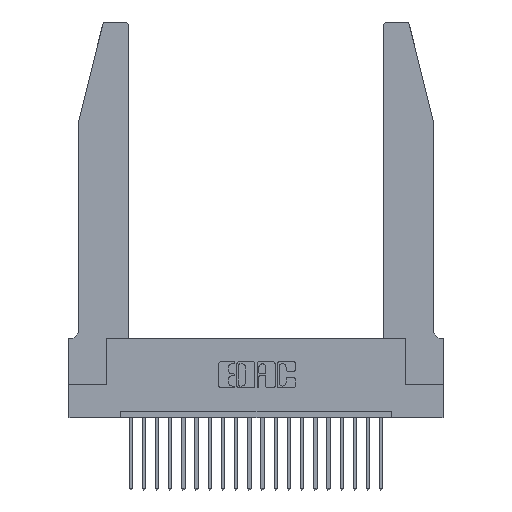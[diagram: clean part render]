
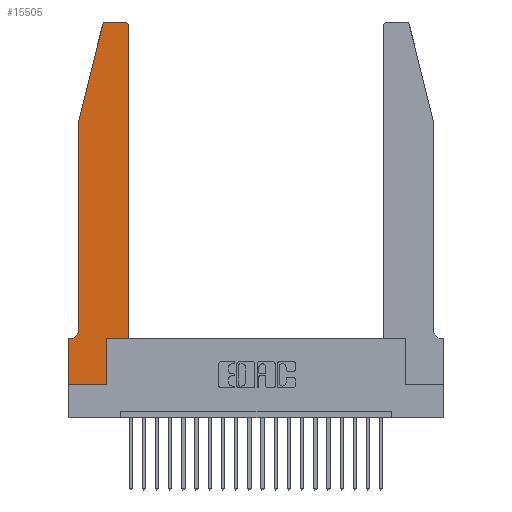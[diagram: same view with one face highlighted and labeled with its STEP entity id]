
A CAD part, top view. The second image highlights one B-rep face of the part: STEP entity #15505.
In plain terms, the highlighted planar face has unit normal (0, 0, 1).
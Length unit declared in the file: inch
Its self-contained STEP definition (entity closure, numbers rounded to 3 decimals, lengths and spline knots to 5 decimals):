
#384 = DIRECTION ( 'NONE',  ( 0., -1., 0. ) ) ;
#406 = CARTESIAN_POINT ( 'NONE',  ( 0.2865, 0.35, 0.37 ) ) ;
#459 = EDGE_CURVE ( 'NONE', #22154, #4561, #3042, .T. ) ;
#637 = VERTEX_POINT ( 'NONE', #22214 ) ;
#841 = DIRECTION ( 'NONE',  ( 0., 0., 1. ) ) ;
#859 = AXIS2_PLACEMENT_3D ( 'NONE', #9379, #18287, #14597 ) ;
#917 = LINE ( 'NONE', #16121, #5352 ) ;
#1115 = LINE ( 'NONE', #6420, #7210 ) ;
#1199 = VERTEX_POINT ( 'NONE', #1847 ) ;
#1201 = ORIENTED_EDGE ( 'NONE', *, *, #12036, .T. ) ;
#1287 = ORIENTED_EDGE ( 'NONE', *, *, #14387, .T. ) ;
#1458 = DIRECTION ( 'NONE',  ( 1., 0., 0. ) ) ;
#1847 = CARTESIAN_POINT ( 'NONE',  ( 0.25487, 2.72718, 0.37 ) ) ;
#2315 = LINE ( 'NONE', #10882, #7547 ) ;
#2342 = VECTOR ( 'NONE', #6219, 39.37008 ) ;
#2479 = ORIENTED_EDGE ( 'NONE', *, *, #12686, .T. ) ;
#2658 = PLANE ( 'NONE',  #859 ) ;
#2955 = CARTESIAN_POINT ( 'NONE',  ( 0.4505, 0.35, 0.37 ) ) ;
#3042 = CIRCLE ( 'NONE', #22489, 0.03 ) ;
#3784 = ORIENTED_EDGE ( 'NONE', *, *, #10910, .T. ) ;
#3871 = VECTOR ( 'NONE', #19753, 39.37008 ) ;
#4238 = DIRECTION ( 'NONE',  ( 0., 1., 0. ) ) ;
#4561 = VERTEX_POINT ( 'NONE', #5781 ) ;
#4858 = VERTEX_POINT ( 'NONE', #21135 ) ;
#4943 = CARTESIAN_POINT ( 'NONE',  ( 0., 0., 0.37 ) ) ;
#4972 = DIRECTION ( 'NONE',  ( 0., 0., -1. ) ) ;
#5352 = VECTOR ( 'NONE', #5683, 39.37008 ) ;
#5404 = DIRECTION ( 'NONE',  ( 1., 0., 0. ) ) ;
#5683 = DIRECTION ( 'NONE',  ( -1., 0., 0. ) ) ;
#5719 = DIRECTION ( 'NONE',  ( 0., 0., 1. ) ) ;
#5781 = CARTESIAN_POINT ( 'NONE',  ( 0.4205, 2.75, 0.37 ) ) ;
#6219 = DIRECTION ( 'NONE',  ( 0., 1., 0. ) ) ;
#6420 = CARTESIAN_POINT ( 'NONE',  ( 0.0755, 2., 0.37 ) ) ;
#6532 = CARTESIAN_POINT ( 'NONE',  ( 0.0055, 0.42, 0.37 ) ) ;
#6735 = VECTOR ( 'NONE', #15798, 39.37008 ) ;
#6936 = EDGE_LOOP ( 'NONE', ( #21626, #1287, #1201, #2479, #14237, #21215, #8851, #3784, #11125, #22543, #9801, #12540 ) ) ;
#7210 = VECTOR ( 'NONE', #9881, 39.37008 ) ;
#7235 = LINE ( 'NONE', #4943, #19530 ) ;
#7547 = VECTOR ( 'NONE', #384, 39.37008 ) ;
#7924 = AXIS2_PLACEMENT_3D ( 'NONE', #6532, #4972, #8370 ) ;
#8034 = CARTESIAN_POINT ( 'NONE',  ( 0.4505, 2.72, 0.37 ) ) ;
#8054 = LINE ( 'NONE', #12281, #20352 ) ;
#8370 = DIRECTION ( 'NONE',  ( -1., 0., 0. ) ) ;
#8851 = ORIENTED_EDGE ( 'NONE', *, *, #16362, .T. ) ;
#9214 = EDGE_CURVE ( 'NONE', #21976, #17296, #9794, .T. ) ;
#9379 = CARTESIAN_POINT ( 'NONE',  ( 0., 0.35, 0.37 ) ) ;
#9600 = EDGE_CURVE ( 'NONE', #4858, #22154, #19035, .T. ) ;
#9701 = VERTEX_POINT ( 'NONE', #17264 ) ;
#9794 = LINE ( 'NONE', #14710, #14934 ) ;
#9801 = ORIENTED_EDGE ( 'NONE', *, *, #9600, .T. ) ;
#9860 = CARTESIAN_POINT ( 'NONE',  ( 0.0755, 0.42, 0.37 ) ) ;
#9881 = DIRECTION ( 'NONE',  ( -0.239, -0.971, 0. ) ) ;
#9922 = EDGE_CURVE ( 'NONE', #14641, #637, #19582, .T. ) ;
#10882 = CARTESIAN_POINT ( 'NONE',  ( 0., 0., 0.37 ) ) ;
#10886 = CARTESIAN_POINT ( 'NONE',  ( 0.2865, 0., 0.37 ) ) ;
#10910 = EDGE_CURVE ( 'NONE', #22359, #21976, #7235, .T. ) ;
#11125 = ORIENTED_EDGE ( 'NONE', *, *, #9214, .T. ) ;
#11634 = AXIS2_PLACEMENT_3D ( 'NONE', #16158, #5719, #17941 ) ;
#11737 = EDGE_CURVE ( 'NONE', #17296, #4858, #8054, .T. ) ;
#12006 = CARTESIAN_POINT ( 'NONE',  ( 0.0755, 2., 0.37 ) ) ;
#12036 = EDGE_CURVE ( 'NONE', #1199, #12834, #1115, .T. ) ;
#12209 = CARTESIAN_POINT ( 'NONE',  ( 0., 0., 0.37 ) ) ;
#12281 = CARTESIAN_POINT ( 'NONE',  ( 0.4505, 0.35, 0.37 ) ) ;
#12540 = ORIENTED_EDGE ( 'NONE', *, *, #459, .T. ) ;
#12686 = EDGE_CURVE ( 'NONE', #12834, #14280, #17003, .T. ) ;
#12834 = VERTEX_POINT ( 'NONE', #12006 ) ;
#12839 = CARTESIAN_POINT ( 'NONE',  ( 0.0755, 2., 0.37 ) ) ;
#14237 = ORIENTED_EDGE ( 'NONE', *, *, #21799, .T. ) ;
#14280 = VERTEX_POINT ( 'NONE', #9860 ) ;
#14384 = FACE_OUTER_BOUND ( 'NONE', #6936, .T. ) ;
#14387 = EDGE_CURVE ( 'NONE', #9701, #1199, #15268, .T. ) ;
#14597 = DIRECTION ( 'NONE',  ( 1., 0., 0. ) ) ;
#14641 = VERTEX_POINT ( 'NONE', #16525 ) ;
#14710 = CARTESIAN_POINT ( 'NONE',  ( 0.2865, 0.35, 0.37 ) ) ;
#14934 = VECTOR ( 'NONE', #4238, 39.37008 ) ;
#15268 = CIRCLE ( 'NONE', #11634, 0.03 ) ;
#15505 = ADVANCED_FACE ( 'NONE', ( #14384 ), #2658, .T. ) ;
#15798 = DIRECTION ( 'NONE',  ( -1., 0., 0. ) ) ;
#15880 = CARTESIAN_POINT ( 'NONE',  ( 0.0755, 0.35, 0.37 ) ) ;
#16059 = EDGE_CURVE ( 'NONE', #4561, #9701, #917, .T. ) ;
#16121 = CARTESIAN_POINT ( 'NONE',  ( 0.2605, 2.75, 0.37 ) ) ;
#16158 = CARTESIAN_POINT ( 'NONE',  ( 0.284, 2.72, 0.37 ) ) ;
#16362 = EDGE_CURVE ( 'NONE', #637, #22359, #2315, .T. ) ;
#16525 = CARTESIAN_POINT ( 'NONE',  ( 0.0055, 0.35, 0.37 ) ) ;
#16794 = CIRCLE ( 'NONE', #7924, 0.07 ) ;
#17003 = LINE ( 'NONE', #12839, #3871 ) ;
#17264 = CARTESIAN_POINT ( 'NONE',  ( 0.284, 2.75, 0.37 ) ) ;
#17296 = VERTEX_POINT ( 'NONE', #406 ) ;
#17941 = DIRECTION ( 'NONE',  ( 1., 0., 0. ) ) ;
#18287 = DIRECTION ( 'NONE',  ( 0., 0., 1. ) ) ;
#19035 = LINE ( 'NONE', #2955, #2342 ) ;
#19530 = VECTOR ( 'NONE', #1458, 39.37008 ) ;
#19582 = LINE ( 'NONE', #15880, #6735 ) ;
#19753 = DIRECTION ( 'NONE',  ( 0., -1., 0. ) ) ;
#20256 = CARTESIAN_POINT ( 'NONE',  ( 0.4205, 2.72, 0.37 ) ) ;
#20352 = VECTOR ( 'NONE', #5404, 39.37008 ) ;
#21135 = CARTESIAN_POINT ( 'NONE',  ( 0.4505, 0.35, 0.37 ) ) ;
#21215 = ORIENTED_EDGE ( 'NONE', *, *, #9922, .T. ) ;
#21626 = ORIENTED_EDGE ( 'NONE', *, *, #16059, .T. ) ;
#21799 = EDGE_CURVE ( 'NONE', #14280, #14641, #16794, .T. ) ;
#21976 = VERTEX_POINT ( 'NONE', #10886 ) ;
#21986 = DIRECTION ( 'NONE',  ( 1., 0., 0. ) ) ;
#22154 = VERTEX_POINT ( 'NONE', #8034 ) ;
#22214 = CARTESIAN_POINT ( 'NONE',  ( 0., 0.35, 0.37 ) ) ;
#22359 = VERTEX_POINT ( 'NONE', #12209 ) ;
#22489 = AXIS2_PLACEMENT_3D ( 'NONE', #20256, #841, #21986 ) ;
#22543 = ORIENTED_EDGE ( 'NONE', *, *, #11737, .T. ) ;
